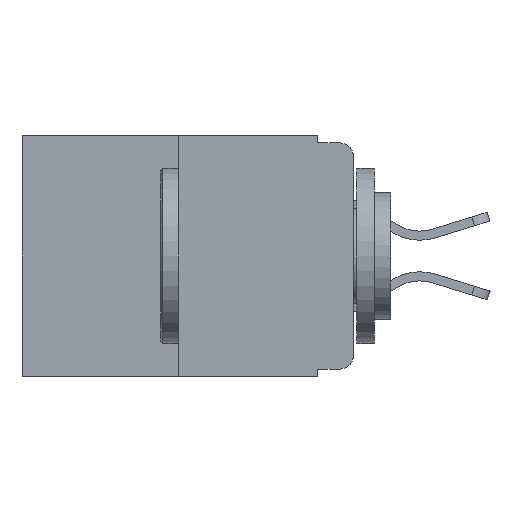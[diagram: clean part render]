
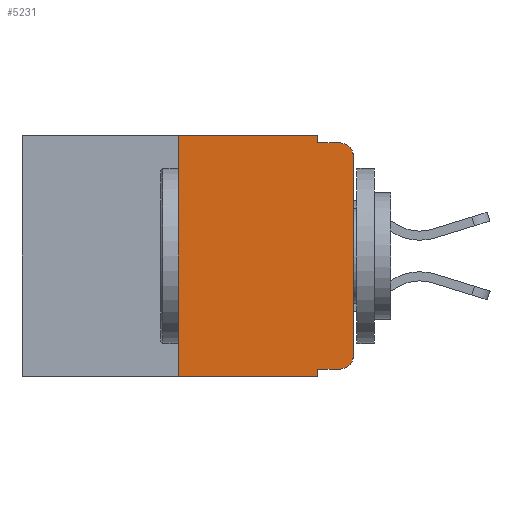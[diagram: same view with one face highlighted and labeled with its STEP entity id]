
A CAD part, left-side view. The second image highlights one B-rep face of the part: STEP entity #5231.
In plain terms, the highlighted planar face has unit normal (-1, 0, 0).
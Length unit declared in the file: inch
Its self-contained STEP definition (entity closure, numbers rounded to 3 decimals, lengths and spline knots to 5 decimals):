
#213 = VERTEX_POINT ( 'NONE', #3985 ) ;
#319 = EDGE_CURVE ( 'NONE', #7232, #6145, #10229, .T. ) ;
#531 = VECTOR ( 'NONE', #11401, 39.37008 ) ;
#535 = EDGE_CURVE ( 'NONE', #4646, #13100, #4570, .T. ) ;
#682 = EDGE_CURVE ( 'NONE', #213, #9471, #12704, .T. ) ;
#740 = AXIS2_PLACEMENT_3D ( 'NONE', #1912, #4040, #11209 ) ;
#762 = DIRECTION ( 'NONE',  ( 0., -1., 0. ) ) ;
#852 = DIRECTION ( 'NONE',  ( -1., 0., 0. ) ) ;
#1242 = EDGE_LOOP ( 'NONE', ( #12808, #10655, #7998, #11586, #4469, #11090, #4229, #8670, #6422, #10723 ) ) ;
#1534 = CARTESIAN_POINT ( 'NONE',  ( 0., 0.051, -0.01 ) ) ;
#1734 = LINE ( 'NONE', #7936, #4664 ) ;
#1753 = VECTOR ( 'NONE', #4706, 39.37008 ) ;
#1848 = LINE ( 'NONE', #5909, #1753 ) ;
#1912 = CARTESIAN_POINT ( 'NONE',  ( 0., 0.02, -0.313 ) ) ;
#2007 = EDGE_CURVE ( 'NONE', #6952, #4646, #4926, .T. ) ;
#3985 = CARTESIAN_POINT ( 'NONE',  ( 0., 0.02, -0.333 ) ) ;
#4040 = DIRECTION ( 'NONE',  ( -1., 0., 0. ) ) ;
#4229 = ORIENTED_EDGE ( 'NONE', *, *, #319, .T. ) ;
#4469 = ORIENTED_EDGE ( 'NONE', *, *, #11559, .F. ) ;
#4570 = LINE ( 'NONE', #8652, #8214 ) ;
#4626 = CARTESIAN_POINT ( 'NONE',  ( 0., 0.051, 0. ) ) ;
#4646 = VERTEX_POINT ( 'NONE', #1534 ) ;
#4664 = VECTOR ( 'NONE', #12762, 39.37008 ) ;
#4697 = EDGE_CURVE ( 'NONE', #7758, #13100, #10013, .T. ) ;
#4706 = DIRECTION ( 'NONE',  ( 0., 0., -1. ) ) ;
#4926 = LINE ( 'NONE', #5253, #5921 ) ;
#4954 = AXIS2_PLACEMENT_3D ( 'NONE', #10807, #10882, #6778 ) ;
#5131 = CARTESIAN_POINT ( 'NONE',  ( 0., 0.473, -0.343 ) ) ;
#5143 = EDGE_CURVE ( 'NONE', #7970, #6145, #1848, .T. ) ;
#5231 = ADVANCED_FACE ( 'NONE', ( #11819 ), #7852, .F. ) ;
#5243 = CARTESIAN_POINT ( 'NONE',  ( 0., 0.25, -0.343 ) ) ;
#5253 = CARTESIAN_POINT ( 'NONE',  ( 0., 0.051, 0. ) ) ;
#5357 = LINE ( 'NONE', #10585, #6123 ) ;
#5544 = DIRECTION ( 'NONE',  ( 0., 0., 1. ) ) ;
#5594 = DIRECTION ( 'NONE',  ( 0., 0., 1. ) ) ;
#5783 = LINE ( 'NONE', #8872, #8745 ) ;
#5909 = CARTESIAN_POINT ( 'NONE',  ( 0., 0.051, 0. ) ) ;
#5921 = VECTOR ( 'NONE', #9021, 39.37008 ) ;
#6123 = VECTOR ( 'NONE', #5544, 39.37008 ) ;
#6145 = VERTEX_POINT ( 'NONE', #12487 ) ;
#6261 = DIRECTION ( 'NONE',  ( 0., -1., 0. ) ) ;
#6287 = CARTESIAN_POINT ( 'NONE',  ( 0., 0., -0.03 ) ) ;
#6422 = ORIENTED_EDGE ( 'NONE', *, *, #7177, .T. ) ;
#6778 = DIRECTION ( 'NONE',  ( 0., 0., -1. ) ) ;
#6952 = VERTEX_POINT ( 'NONE', #4626 ) ;
#7076 = CARTESIAN_POINT ( 'NONE',  ( 0., 0.02, -0.01 ) ) ;
#7177 = EDGE_CURVE ( 'NONE', #7970, #213, #9072, .T. ) ;
#7232 = VERTEX_POINT ( 'NONE', #5243 ) ;
#7559 = VECTOR ( 'NONE', #6261, 39.37008 ) ;
#7758 = VERTEX_POINT ( 'NONE', #6287 ) ;
#7852 = PLANE ( 'NONE',  #4954 ) ;
#7936 = CARTESIAN_POINT ( 'NONE',  ( 0., 0.473, 0. ) ) ;
#7970 = VERTEX_POINT ( 'NONE', #10832 ) ;
#7998 = ORIENTED_EDGE ( 'NONE', *, *, #535, .F. ) ;
#8214 = VECTOR ( 'NONE', #762, 39.37008 ) ;
#8652 = CARTESIAN_POINT ( 'NONE',  ( 0., 0.051, -0.01 ) ) ;
#8670 = ORIENTED_EDGE ( 'NONE', *, *, #5143, .F. ) ;
#8745 = VECTOR ( 'NONE', #5594, 39.37008 ) ;
#8872 = CARTESIAN_POINT ( 'NONE',  ( 0., 0.25, 0. ) ) ;
#8873 = VERTEX_POINT ( 'NONE', #10613 ) ;
#9021 = DIRECTION ( 'NONE',  ( 0., 0., -1. ) ) ;
#9067 = EDGE_CURVE ( 'NONE', #9471, #7758, #5357, .T. ) ;
#9072 = LINE ( 'NONE', #13135, #531 ) ;
#9471 = VERTEX_POINT ( 'NONE', #11632 ) ;
#9590 = AXIS2_PLACEMENT_3D ( 'NONE', #12898, #852, #13093 ) ;
#10013 = CIRCLE ( 'NONE', #9590, 0.02 ) ;
#10229 = LINE ( 'NONE', #5131, #7559 ) ;
#10585 = CARTESIAN_POINT ( 'NONE',  ( 0., 0., 0. ) ) ;
#10613 = CARTESIAN_POINT ( 'NONE',  ( 0., 0.25, 0. ) ) ;
#10655 = ORIENTED_EDGE ( 'NONE', *, *, #4697, .T. ) ;
#10723 = ORIENTED_EDGE ( 'NONE', *, *, #682, .T. ) ;
#10807 = CARTESIAN_POINT ( 'NONE',  ( 0., 0.473, 0. ) ) ;
#10832 = CARTESIAN_POINT ( 'NONE',  ( 0., 0.051, -0.333 ) ) ;
#10882 = DIRECTION ( 'NONE',  ( 1., 0., 0. ) ) ;
#11090 = ORIENTED_EDGE ( 'NONE', *, *, #11943, .F. ) ;
#11209 = DIRECTION ( 'NONE',  ( 0., 0., -1. ) ) ;
#11401 = DIRECTION ( 'NONE',  ( 0., -1., 0. ) ) ;
#11559 = EDGE_CURVE ( 'NONE', #8873, #6952, #1734, .T. ) ;
#11586 = ORIENTED_EDGE ( 'NONE', *, *, #2007, .F. ) ;
#11632 = CARTESIAN_POINT ( 'NONE',  ( 0., 0., -0.313 ) ) ;
#11819 = FACE_OUTER_BOUND ( 'NONE', #1242, .T. ) ;
#11943 = EDGE_CURVE ( 'NONE', #7232, #8873, #5783, .T. ) ;
#12487 = CARTESIAN_POINT ( 'NONE',  ( 0., 0.051, -0.343 ) ) ;
#12704 = CIRCLE ( 'NONE', #740, 0.02 ) ;
#12762 = DIRECTION ( 'NONE',  ( 0., -1., 0. ) ) ;
#12808 = ORIENTED_EDGE ( 'NONE', *, *, #9067, .T. ) ;
#12898 = CARTESIAN_POINT ( 'NONE',  ( 0., 0.02, -0.03 ) ) ;
#13093 = DIRECTION ( 'NONE',  ( 0., 0., -1. ) ) ;
#13100 = VERTEX_POINT ( 'NONE', #7076 ) ;
#13135 = CARTESIAN_POINT ( 'NONE',  ( 0., 0.051, -0.333 ) ) ;
